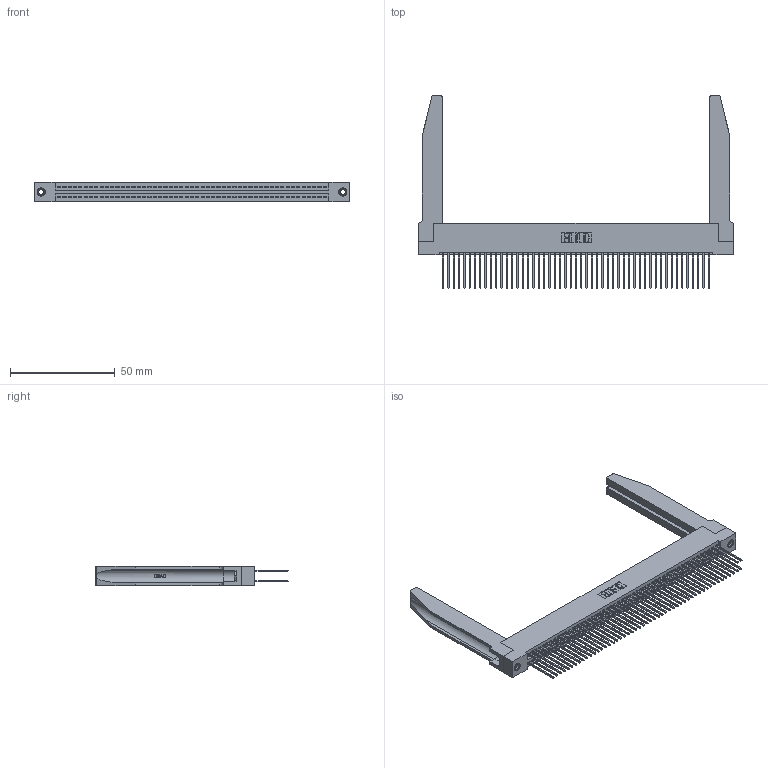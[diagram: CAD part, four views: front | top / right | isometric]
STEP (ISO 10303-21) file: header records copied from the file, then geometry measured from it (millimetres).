
FILE_DESCRIPTION (( 'STEP AP203' ), '1' );
FILE_NAME ('345-102-542-278.STEP', '2019-11-03T08:14:25', ( '' ), ( '' ), 'SwSTEP 2.0', 'SolidWorks 2016', '' );
FILE_SCHEMA (( 'CONFIG_CONTROL_DESIGN' ));
Length unit declared in the file: inch
Products named in the file (5): 345-292-001_345-293-142; 345-250-001_345-250-001-102; 345-220-078_345-220-078; 345 Part_Flush Mounting Lugs - 0.156 Dia-TH; 345-102-542-278
Assembly tree (107 placements, depth 2):
  345-102-542-278
    345 Part_Flush Mounting Lugs - 0.156 Dia-TH
    345-292-001_345-293-142  x102
    345-250-001_345-250-001-102  x2
    345-220-078_345-220-078  x2
Bounding box: 150.77 x 92.25 x 9.4 mm (x, y, z)
Volume: 22975.8 mm3; surface area: 31711 mm2
Topology: 107 solids, 107 shells, 5460 faces, 16147 edges, 10618 vertices
Faces by surface type: plane 3588, cylinder 1820, bspline 36, cone 12, torus 4
Entity records: 43562 total; most frequent: CARTESIAN_POINT 8211, ORIENTED_EDGE 7042, DIRECTION 6223, EDGE_CURVE 3521, LINE 3091, VECTOR 3091, VERTEX_POINT 2340, AXIS2_PLACEMENT_3D 1566
